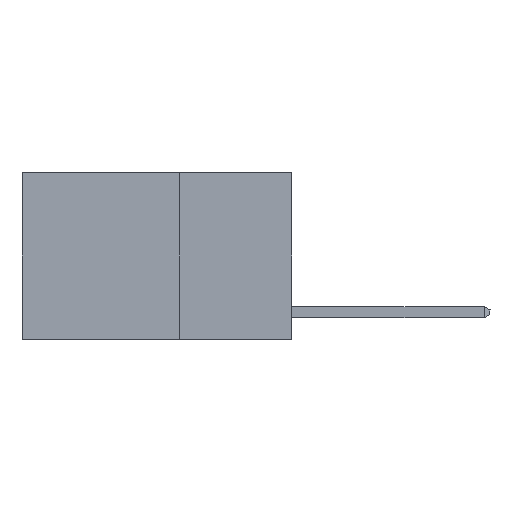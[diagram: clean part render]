
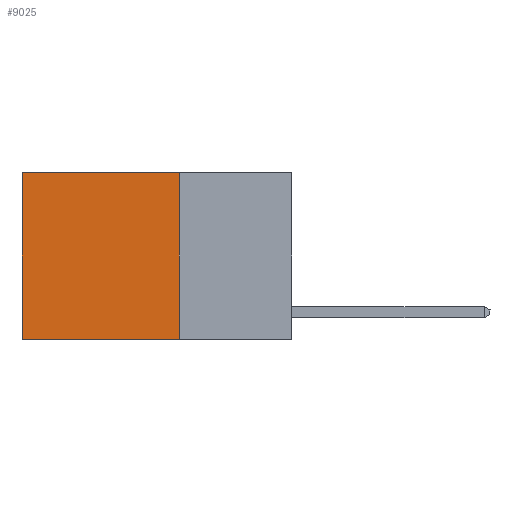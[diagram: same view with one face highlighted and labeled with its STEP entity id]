
A CAD part, left-side view. The second image highlights one B-rep face of the part: STEP entity #9025.
In plain terms, the highlighted planar face has unit normal (-1, 0, 0).
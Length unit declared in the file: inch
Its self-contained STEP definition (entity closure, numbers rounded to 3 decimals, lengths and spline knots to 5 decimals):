
#1342 = VECTOR ( 'NONE', #17460, 39.37008 ) ;
#1624 = DIRECTION ( 'NONE',  ( 0., 0., -1. ) ) ;
#1871 = EDGE_CURVE ( 'NONE', #2756, #2433, #11559, .T. ) ;
#1988 = CARTESIAN_POINT ( 'NONE',  ( 0.2625, 0.25, 0. ) ) ;
#2058 = CARTESIAN_POINT ( 'NONE',  ( 0.2625, 0.25, -0.37 ) ) ;
#2162 = ORIENTED_EDGE ( 'NONE', *, *, #12806, .T. ) ;
#2250 = ORIENTED_EDGE ( 'NONE', *, *, #1871, .T. ) ;
#2433 = VERTEX_POINT ( 'NONE', #5018 ) ;
#2756 = VERTEX_POINT ( 'NONE', #12885 ) ;
#3380 = CARTESIAN_POINT ( 'NONE',  ( 0.2625, 0.25, 0. ) ) ;
#4180 = VERTEX_POINT ( 'NONE', #2058 ) ;
#4769 = FACE_OUTER_BOUND ( 'NONE', #17702, .T. ) ;
#5018 = CARTESIAN_POINT ( 'NONE',  ( 0.2625, 0.6, 0. ) ) ;
#5592 = ORIENTED_EDGE ( 'NONE', *, *, #8152, .F. ) ;
#5935 = AXIS2_PLACEMENT_3D ( 'NONE', #3380, #15966, #7648 ) ;
#6049 = CARTESIAN_POINT ( 'NONE',  ( 0.2625, 0.25, 0. ) ) ;
#6359 = DIRECTION ( 'NONE',  ( 0., 1., 0. ) ) ;
#6668 = VECTOR ( 'NONE', #1624, 39.37008 ) ;
#7350 = VERTEX_POINT ( 'NONE', #9435 ) ;
#7648 = DIRECTION ( 'NONE',  ( 0., 0., -1. ) ) ;
#7741 = ORIENTED_EDGE ( 'NONE', *, *, #14588, .F. ) ;
#8152 = EDGE_CURVE ( 'NONE', #4180, #7350, #16087, .T. ) ;
#8440 = CARTESIAN_POINT ( 'NONE',  ( 0.2625, 0.6, 0. ) ) ;
#9025 = ADVANCED_FACE ( 'NONE', ( #4769 ), #13017, .F. ) ;
#9435 = CARTESIAN_POINT ( 'NONE',  ( 0.2625, 0.6, -0.37 ) ) ;
#10718 = VECTOR ( 'NONE', #11038, 39.37008 ) ;
#11038 = DIRECTION ( 'NONE',  ( 0., 0., -1. ) ) ;
#11541 = LINE ( 'NONE', #1988, #6668 ) ;
#11559 = LINE ( 'NONE', #6049, #1342 ) ;
#12127 = CARTESIAN_POINT ( 'NONE',  ( 0.2625, 0.25, -0.37 ) ) ;
#12806 = EDGE_CURVE ( 'NONE', #2433, #7350, #18231, .T. ) ;
#12885 = CARTESIAN_POINT ( 'NONE',  ( 0.2625, 0.25, 0. ) ) ;
#13017 = PLANE ( 'NONE',  #5935 ) ;
#14588 = EDGE_CURVE ( 'NONE', #2756, #4180, #11541, .T. ) ;
#15966 = DIRECTION ( 'NONE',  ( 1., 0., 0. ) ) ;
#16087 = LINE ( 'NONE', #12127, #17515 ) ;
#17460 = DIRECTION ( 'NONE',  ( 0., 1., 0. ) ) ;
#17515 = VECTOR ( 'NONE', #6359, 39.37008 ) ;
#17702 = EDGE_LOOP ( 'NONE', ( #2162, #5592, #7741, #2250 ) ) ;
#18231 = LINE ( 'NONE', #8440, #10718 ) ;
